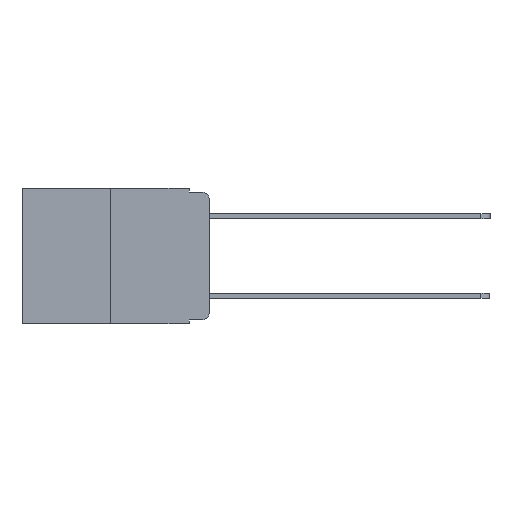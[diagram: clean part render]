
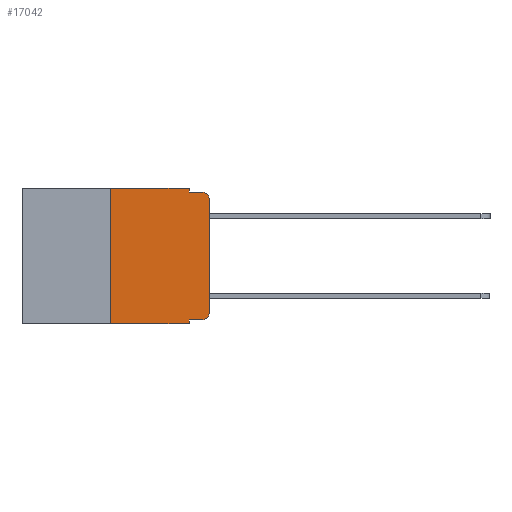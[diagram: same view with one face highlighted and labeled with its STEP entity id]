
A CAD part, left-side view. The second image highlights one B-rep face of the part: STEP entity #17042.
In plain terms, the highlighted planar face has unit normal (-1, 0, 0).
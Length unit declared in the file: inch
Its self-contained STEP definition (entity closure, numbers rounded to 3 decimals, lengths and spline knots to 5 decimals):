
#11 = EDGE_CURVE ( 'NONE', #6556, #1439, #4447, .T. ) ;
#897 = EDGE_CURVE ( 'NONE', #1439, #4785, #9246, .T. ) ;
#931 = VECTOR ( 'NONE', #9401, 39.37008 ) ;
#937 = DIRECTION ( 'NONE',  ( 0., 0., -1. ) ) ;
#1119 = CARTESIAN_POINT ( 'NONE',  ( 0., 0., 0. ) ) ;
#1187 = CARTESIAN_POINT ( 'NONE',  ( 0., 0.25, -0.343 ) ) ;
#1284 = CARTESIAN_POINT ( 'NONE',  ( 0., 0.051, -0.01 ) ) ;
#1439 = VERTEX_POINT ( 'NONE', #7747 ) ;
#1493 = VERTEX_POINT ( 'NONE', #2792 ) ;
#1736 = EDGE_CURVE ( 'NONE', #12971, #1493, #14408, .T. ) ;
#2095 = EDGE_CURVE ( 'NONE', #17269, #3427, #4625, .T. ) ;
#2389 = CARTESIAN_POINT ( 'NONE',  ( 0., 0.051, -0.333 ) ) ;
#2702 = EDGE_CURVE ( 'NONE', #16677, #12971, #10077, .T. ) ;
#2716 = CARTESIAN_POINT ( 'NONE',  ( 0., 0., -0.313 ) ) ;
#2792 = CARTESIAN_POINT ( 'NONE',  ( 0., 0.02, -0.01 ) ) ;
#2825 = VERTEX_POINT ( 'NONE', #5438 ) ;
#3427 = VERTEX_POINT ( 'NONE', #8062 ) ;
#3702 = DIRECTION ( 'NONE',  ( 1., 0., 0. ) ) ;
#3764 = VECTOR ( 'NONE', #10616, 39.37008 ) ;
#4089 = EDGE_CURVE ( 'NONE', #15390, #6556, #9411, .T. ) ;
#4312 = DIRECTION ( 'NONE',  ( 0., 0., 1. ) ) ;
#4434 = EDGE_CURVE ( 'NONE', #17269, #2825, #10658, .T. ) ;
#4447 = LINE ( 'NONE', #13932, #7579 ) ;
#4625 = LINE ( 'NONE', #15979, #931 ) ;
#4785 = VERTEX_POINT ( 'NONE', #8546 ) ;
#5438 = CARTESIAN_POINT ( 'NONE',  ( 0., 0.051, -0.343 ) ) ;
#5620 = DIRECTION ( 'NONE',  ( -1., 0., 0. ) ) ;
#5650 = VECTOR ( 'NONE', #16587, 39.37008 ) ;
#6469 = EDGE_CURVE ( 'NONE', #15390, #2825, #13906, .T. ) ;
#6556 = VERTEX_POINT ( 'NONE', #13820 ) ;
#6934 = ORIENTED_EDGE ( 'NONE', *, *, #1736, .T. ) ;
#7296 = DIRECTION ( 'NONE',  ( -1., 0., 0. ) ) ;
#7503 = ORIENTED_EDGE ( 'NONE', *, *, #897, .F. ) ;
#7579 = VECTOR ( 'NONE', #8596, 39.37008 ) ;
#7747 = CARTESIAN_POINT ( 'NONE',  ( 0., 0.051, 0. ) ) ;
#7920 = ORIENTED_EDGE ( 'NONE', *, *, #2095, .T. ) ;
#8020 = ORIENTED_EDGE ( 'NONE', *, *, #11470, .F. ) ;
#8062 = CARTESIAN_POINT ( 'NONE',  ( 0., 0.02, -0.333 ) ) ;
#8071 = DIRECTION ( 'NONE',  ( 0., -1., 0. ) ) ;
#8160 = ORIENTED_EDGE ( 'NONE', *, *, #2702, .T. ) ;
#8465 = AXIS2_PLACEMENT_3D ( 'NONE', #11735, #3702, #13097 ) ;
#8546 = CARTESIAN_POINT ( 'NONE',  ( 0., 0.051, -0.01 ) ) ;
#8596 = DIRECTION ( 'NONE',  ( 0., -1., 0. ) ) ;
#8753 = ORIENTED_EDGE ( 'NONE', *, *, #11, .F. ) ;
#8770 = ORIENTED_EDGE ( 'NONE', *, *, #4089, .F. ) ;
#8959 = AXIS2_PLACEMENT_3D ( 'NONE', #13670, #5620, #14968 ) ;
#9038 = ORIENTED_EDGE ( 'NONE', *, *, #4434, .F. ) ;
#9117 = ORIENTED_EDGE ( 'NONE', *, *, #10383, .T. ) ;
#9190 = ORIENTED_EDGE ( 'NONE', *, *, #6469, .T. ) ;
#9246 = LINE ( 'NONE', #13276, #5650 ) ;
#9401 = DIRECTION ( 'NONE',  ( 0., -1., 0. ) ) ;
#9411 = LINE ( 'NONE', #13674, #16796 ) ;
#10077 = LINE ( 'NONE', #1119, #3764 ) ;
#10383 = EDGE_CURVE ( 'NONE', #3427, #16677, #11667, .T. ) ;
#10446 = CARTESIAN_POINT ( 'NONE',  ( 0., 0.051, 0. ) ) ;
#10616 = DIRECTION ( 'NONE',  ( 0., 0., 1. ) ) ;
#10658 = LINE ( 'NONE', #10446, #13784 ) ;
#11280 = CARTESIAN_POINT ( 'NONE',  ( 0., 0., -0.03 ) ) ;
#11470 = EDGE_CURVE ( 'NONE', #4785, #1493, #13454, .T. ) ;
#11667 = CIRCLE ( 'NONE', #8959, 0.02 ) ;
#11735 = CARTESIAN_POINT ( 'NONE',  ( 0., 0.473, 0. ) ) ;
#12875 = FACE_OUTER_BOUND ( 'NONE', #15034, .T. ) ;
#12971 = VERTEX_POINT ( 'NONE', #11280 ) ;
#13097 = DIRECTION ( 'NONE',  ( 0., 0., -1. ) ) ;
#13276 = CARTESIAN_POINT ( 'NONE',  ( 0., 0.051, 0. ) ) ;
#13454 = LINE ( 'NONE', #1284, #16464 ) ;
#13670 = CARTESIAN_POINT ( 'NONE',  ( 0., 0.02, -0.313 ) ) ;
#13674 = CARTESIAN_POINT ( 'NONE',  ( 0., 0.25, 0. ) ) ;
#13784 = VECTOR ( 'NONE', #937, 39.37008 ) ;
#13820 = CARTESIAN_POINT ( 'NONE',  ( 0., 0.25, 0. ) ) ;
#13906 = LINE ( 'NONE', #14962, #16514 ) ;
#13932 = CARTESIAN_POINT ( 'NONE',  ( 0., 0.473, 0. ) ) ;
#14335 = PLANE ( 'NONE',  #8465 ) ;
#14408 = CIRCLE ( 'NONE', #15808, 0.02 ) ;
#14901 = DIRECTION ( 'NONE',  ( 0., -1., 0. ) ) ;
#14962 = CARTESIAN_POINT ( 'NONE',  ( 0., 0.473, -0.343 ) ) ;
#14968 = DIRECTION ( 'NONE',  ( 0., 0., -1. ) ) ;
#15034 = EDGE_LOOP ( 'NONE', ( #8160, #6934, #8020, #7503, #8753, #8770, #9190, #9038, #7920, #9117 ) ) ;
#15274 = CARTESIAN_POINT ( 'NONE',  ( 0., 0.02, -0.03 ) ) ;
#15390 = VERTEX_POINT ( 'NONE', #1187 ) ;
#15808 = AXIS2_PLACEMENT_3D ( 'NONE', #15274, #7296, #16536 ) ;
#15979 = CARTESIAN_POINT ( 'NONE',  ( 0., 0.051, -0.333 ) ) ;
#16464 = VECTOR ( 'NONE', #8071, 39.37008 ) ;
#16514 = VECTOR ( 'NONE', #14901, 39.37008 ) ;
#16536 = DIRECTION ( 'NONE',  ( 0., 0., -1. ) ) ;
#16587 = DIRECTION ( 'NONE',  ( 0., 0., -1. ) ) ;
#16677 = VERTEX_POINT ( 'NONE', #2716 ) ;
#16796 = VECTOR ( 'NONE', #4312, 39.37008 ) ;
#17042 = ADVANCED_FACE ( 'NONE', ( #12875 ), #14335, .F. ) ;
#17269 = VERTEX_POINT ( 'NONE', #2389 ) ;
